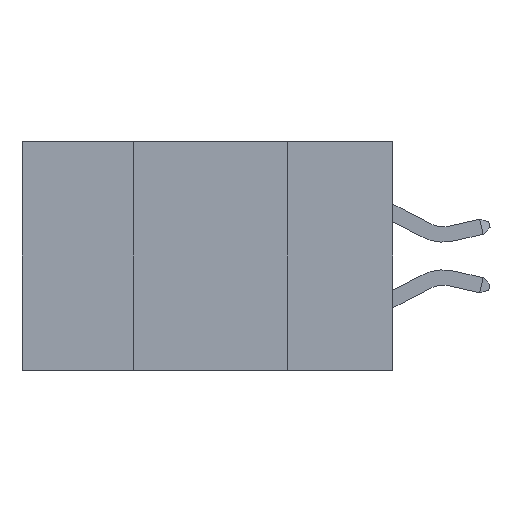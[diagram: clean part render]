
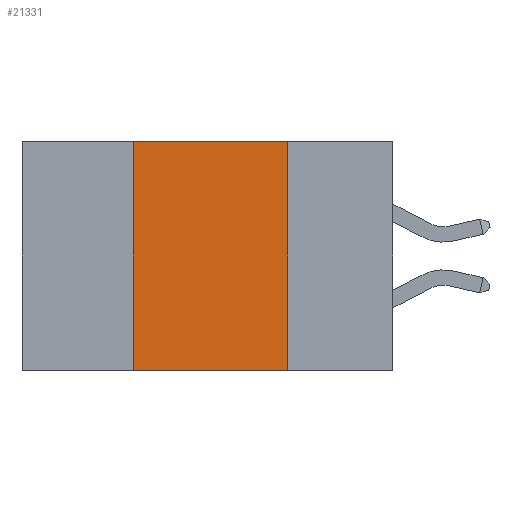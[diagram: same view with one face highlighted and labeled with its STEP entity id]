
A CAD part, left-side view. The second image highlights one B-rep face of the part: STEP entity #21331.
In plain terms, the highlighted planar face has unit normal (-1, 0, 0).
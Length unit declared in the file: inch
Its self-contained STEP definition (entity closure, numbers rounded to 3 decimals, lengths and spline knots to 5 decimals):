
#154 = DIRECTION ( 'NONE',  ( 0., -1., 0. ) ) ;
#1218 = AXIS2_PLACEMENT_3D ( 'NONE', #35469, #10992, #7993 ) ;
#3050 = ORIENTED_EDGE ( 'NONE', *, *, #9415, .F. ) ;
#3176 = CARTESIAN_POINT ( 'NONE',  ( 0., 0.17, 0. ) ) ;
#6095 = CARTESIAN_POINT ( 'NONE',  ( 0., 0.6, -0.37 ) ) ;
#7993 = DIRECTION ( 'NONE',  ( 0., 0., -1. ) ) ;
#8108 = EDGE_CURVE ( 'NONE', #20485, #33442, #18583, .T. ) ;
#9415 = EDGE_CURVE ( 'NONE', #33442, #37056, #24225, .T. ) ;
#10992 = DIRECTION ( 'NONE',  ( 1., 0., 0. ) ) ;
#11381 = FACE_OUTER_BOUND ( 'NONE', #33635, .T. ) ;
#12053 = ORIENTED_EDGE ( 'NONE', *, *, #21107, .F. ) ;
#12513 = LINE ( 'NONE', #6095, #32557 ) ;
#14131 = VECTOR ( 'NONE', #154, 39.37008 ) ;
#16318 = CARTESIAN_POINT ( 'NONE',  ( 0., 0.17, -0.37 ) ) ;
#18355 = EDGE_CURVE ( 'NONE', #20485, #28777, #12513, .T. ) ;
#18385 = ORIENTED_EDGE ( 'NONE', *, *, #18355, .T. ) ;
#18387 = CARTESIAN_POINT ( 'NONE',  ( 0., 0.42, 0. ) ) ;
#18583 = LINE ( 'NONE', #18387, #22303 ) ;
#20485 = VERTEX_POINT ( 'NONE', #23667 ) ;
#21107 = EDGE_CURVE ( 'NONE', #37056, #28777, #35059, .T. ) ;
#21331 = ADVANCED_FACE ( 'NONE', ( #11381 ), #26809, .F. ) ;
#22225 = CARTESIAN_POINT ( 'NONE',  ( 0., 0.17, 0. ) ) ;
#22303 = VECTOR ( 'NONE', #24210, 39.37008 ) ;
#22422 = DIRECTION ( 'NONE',  ( 0., 0., -1. ) ) ;
#23667 = CARTESIAN_POINT ( 'NONE',  ( 0., 0.42, -0.37 ) ) ;
#24210 = DIRECTION ( 'NONE',  ( 0., 0., 1. ) ) ;
#24225 = LINE ( 'NONE', #36458, #14131 ) ;
#26809 = PLANE ( 'NONE',  #1218 ) ;
#28777 = VERTEX_POINT ( 'NONE', #16318 ) ;
#32557 = VECTOR ( 'NONE', #39577, 39.37008 ) ;
#33442 = VERTEX_POINT ( 'NONE', #35776 ) ;
#33635 = EDGE_LOOP ( 'NONE', ( #12053, #3050, #36237, #18385 ) ) ;
#35059 = LINE ( 'NONE', #22225, #35829 ) ;
#35469 = CARTESIAN_POINT ( 'NONE',  ( 0., 0.6, 0. ) ) ;
#35776 = CARTESIAN_POINT ( 'NONE',  ( 0., 0.42, 0. ) ) ;
#35829 = VECTOR ( 'NONE', #22422, 39.37008 ) ;
#36237 = ORIENTED_EDGE ( 'NONE', *, *, #8108, .F. ) ;
#36458 = CARTESIAN_POINT ( 'NONE',  ( 0., 0.6, 0. ) ) ;
#37056 = VERTEX_POINT ( 'NONE', #3176 ) ;
#39577 = DIRECTION ( 'NONE',  ( 0., -1., 0. ) ) ;
